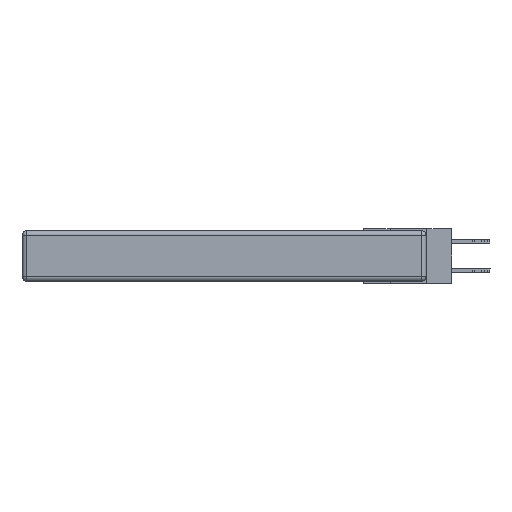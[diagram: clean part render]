
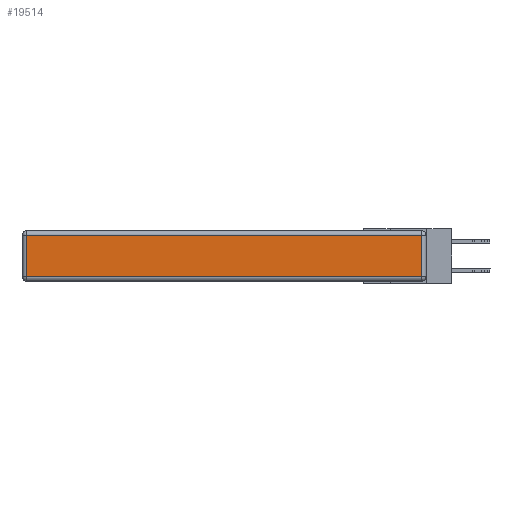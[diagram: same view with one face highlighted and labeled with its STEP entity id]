
A CAD part, left-side view. The second image highlights one B-rep face of the part: STEP entity #19514.
In plain terms, the highlighted planar face has unit normal (-1, 0, 0).
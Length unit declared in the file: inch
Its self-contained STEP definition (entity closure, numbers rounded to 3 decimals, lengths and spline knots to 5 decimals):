
#159 = ORIENTED_EDGE ( 'NONE', *, *, #11832, .T. ) ;
#254 = DIRECTION ( 'NONE',  ( 0., 0., 1. ) ) ;
#314 = VECTOR ( 'NONE', #10119, 39.37008 ) ;
#2359 = PLANE ( 'NONE',  #13026 ) ;
#4109 = CARTESIAN_POINT ( 'NONE',  ( 0., 0.03, -0.343 ) ) ;
#4167 = EDGE_LOOP ( 'NONE', ( #28932, #21438, #159, #14250 ) ) ;
#4809 = CARTESIAN_POINT ( 'NONE',  ( 0., 2.72, -0.343 ) ) ;
#6328 = VECTOR ( 'NONE', #7076, 39.37008 ) ;
#7076 = DIRECTION ( 'NONE',  ( 0., 0., -1. ) ) ;
#7162 = LINE ( 'NONE', #4109, #14419 ) ;
#7896 = CARTESIAN_POINT ( 'NONE',  ( 0., 2.72, -0.03 ) ) ;
#7904 = CARTESIAN_POINT ( 'NONE',  ( 0., 0., -0.313 ) ) ;
#10119 = DIRECTION ( 'NONE',  ( 0., -1., 0. ) ) ;
#11461 = EDGE_CURVE ( 'NONE', #17222, #21717, #21972, .T. ) ;
#11832 = EDGE_CURVE ( 'NONE', #12365, #17222, #16843, .T. ) ;
#12365 = VERTEX_POINT ( 'NONE', #20972 ) ;
#12608 = EDGE_CURVE ( 'NONE', #21717, #26871, #12777, .T. ) ;
#12777 = LINE ( 'NONE', #7904, #314 ) ;
#13026 = AXIS2_PLACEMENT_3D ( 'NONE', #28213, #14107, #254 ) ;
#14107 = DIRECTION ( 'NONE',  ( -1., 0., 0. ) ) ;
#14250 = ORIENTED_EDGE ( 'NONE', *, *, #11461, .T. ) ;
#14419 = VECTOR ( 'NONE', #22831, 39.37008 ) ;
#16584 = CARTESIAN_POINT ( 'NONE',  ( 0., 2.72, -0.313 ) ) ;
#16843 = LINE ( 'NONE', #28008, #22321 ) ;
#17222 = VERTEX_POINT ( 'NONE', #7896 ) ;
#17590 = EDGE_CURVE ( 'NONE', #26871, #12365, #7162, .T. ) ;
#18744 = DIRECTION ( 'NONE',  ( 0., 1., 0. ) ) ;
#19514 = ADVANCED_FACE ( 'NONE', ( #20108 ), #2359, .T. ) ;
#20108 = FACE_OUTER_BOUND ( 'NONE', #4167, .T. ) ;
#20972 = CARTESIAN_POINT ( 'NONE',  ( 0., 0.03, -0.03 ) ) ;
#21438 = ORIENTED_EDGE ( 'NONE', *, *, #17590, .T. ) ;
#21717 = VERTEX_POINT ( 'NONE', #16584 ) ;
#21972 = LINE ( 'NONE', #4809, #6328 ) ;
#22321 = VECTOR ( 'NONE', #18744, 39.37008 ) ;
#22831 = DIRECTION ( 'NONE',  ( 0., 0., 1. ) ) ;
#24357 = CARTESIAN_POINT ( 'NONE',  ( 0., 0.03, -0.313 ) ) ;
#26871 = VERTEX_POINT ( 'NONE', #24357 ) ;
#28008 = CARTESIAN_POINT ( 'NONE',  ( 0., 2.75, -0.03 ) ) ;
#28213 = CARTESIAN_POINT ( 'NONE',  ( 0., 0., -0.343 ) ) ;
#28932 = ORIENTED_EDGE ( 'NONE', *, *, #12608, .T. ) ;
